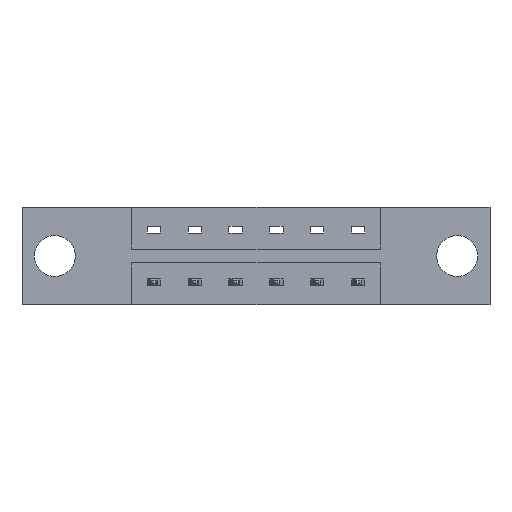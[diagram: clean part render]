
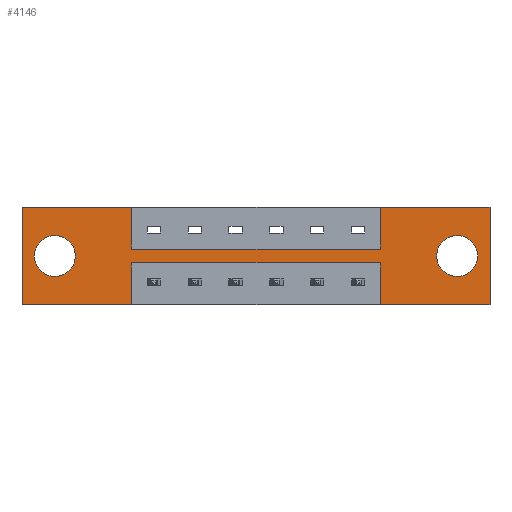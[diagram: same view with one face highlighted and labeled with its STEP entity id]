
A CAD part, front view. The second image highlights one B-rep face of the part: STEP entity #4146.
In plain terms, the highlighted planar face has unit normal (0, -1, 0).
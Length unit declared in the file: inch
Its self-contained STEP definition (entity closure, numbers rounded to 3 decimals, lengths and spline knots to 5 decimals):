
#99 = LINE ( 'NONE', #126, #4949 ) ;
#100 = DIRECTION ( 'NONE',  ( 0., 0., 1. ) ) ;
#126 = CARTESIAN_POINT ( 'NONE',  ( 1.3665, 0., -0.2115 ) ) ;
#155 = DIRECTION ( 'NONE',  ( 0., 0., 1. ) ) ;
#167 = VECTOR ( 'NONE', #100, 39.37008 ) ;
#278 = ORIENTED_EDGE ( 'NONE', *, *, #4959, .T. ) ;
#288 = CARTESIAN_POINT ( 'NONE',  ( 1.3665, 0., 0. ) ) ;
#317 = PLANE ( 'NONE',  #1604 ) ;
#338 = VECTOR ( 'NONE', #7454, 39.37008 ) ;
#372 = EDGE_CURVE ( 'NONE', #6949, #3484, #2396, .T. ) ;
#422 = EDGE_CURVE ( 'NONE', #7205, #1495, #5241, .T. ) ;
#458 = CARTESIAN_POINT ( 'NONE',  ( 0.4175, 0., -0.37 ) ) ;
#490 = EDGE_CURVE ( 'NONE', #2468, #7711, #6305, .T. ) ;
#650 = VERTEX_POINT ( 'NONE', #3517 ) ;
#700 = DIRECTION ( 'NONE',  ( 1., 0., 0. ) ) ;
#738 = EDGE_LOOP ( 'NONE', ( #4732, #3456 ) ) ;
#781 = DIRECTION ( 'NONE',  ( 0., 1., 0. ) ) ;
#785 = LINE ( 'NONE', #6938, #3924 ) ;
#843 = VECTOR ( 'NONE', #6779, 39.37008 ) ;
#920 = VECTOR ( 'NONE', #700, 39.37008 ) ;
#968 = VECTOR ( 'NONE', #1277, 39.37008 ) ;
#1149 = ORIENTED_EDGE ( 'NONE', *, *, #7257, .F. ) ;
#1171 = DIRECTION ( 'NONE',  ( 0., 1., 0. ) ) ;
#1260 = ORIENTED_EDGE ( 'NONE', *, *, #8287, .F. ) ;
#1277 = DIRECTION ( 'NONE',  ( -1., 0., 0. ) ) ;
#1366 = AXIS2_PLACEMENT_3D ( 'NONE', #3649, #3646, #3790 ) ;
#1377 = ORIENTED_EDGE ( 'NONE', *, *, #3852, .F. ) ;
#1420 = EDGE_CURVE ( 'NONE', #1495, #4481, #8238, .T. ) ;
#1432 = DIRECTION ( 'NONE',  ( 1., 0., 0. ) ) ;
#1477 = CARTESIAN_POINT ( 'NONE',  ( 0., 0., -0.37 ) ) ;
#1479 = ORIENTED_EDGE ( 'NONE', *, *, #7361, .F. ) ;
#1495 = VERTEX_POINT ( 'NONE', #5935 ) ;
#1552 = CIRCLE ( 'NONE', #5682, 0.078 ) ;
#1553 = AXIS2_PLACEMENT_3D ( 'NONE', #5091, #1171, #5745 ) ;
#1584 = ORIENTED_EDGE ( 'NONE', *, *, #4797, .F. ) ;
#1604 = AXIS2_PLACEMENT_3D ( 'NONE', #3143, #6990, #3573 ) ;
#1618 = CARTESIAN_POINT ( 'NONE',  ( 0.4175, 0., -0.1585 ) ) ;
#1636 = EDGE_CURVE ( 'NONE', #650, #2468, #7103, .T. ) ;
#1639 = VERTEX_POINT ( 'NONE', #3883 ) ;
#1642 = FACE_BOUND ( 'NONE', #7378, .T. ) ;
#1691 = EDGE_CURVE ( 'NONE', #3484, #6949, #1552, .T. ) ;
#1788 = ORIENTED_EDGE ( 'NONE', *, *, #3382, .F. ) ;
#2017 = CARTESIAN_POINT ( 'NONE',  ( 1.3665, 0., -0.2115 ) ) ;
#2110 = CARTESIAN_POINT ( 'NONE',  ( 0., 0., 0. ) ) ;
#2114 = ORIENTED_EDGE ( 'NONE', *, *, #7131, .F. ) ;
#2246 = AXIS2_PLACEMENT_3D ( 'NONE', #4728, #781, #5379 ) ;
#2396 = CIRCLE ( 'NONE', #1366, 0.078 ) ;
#2468 = VERTEX_POINT ( 'NONE', #288 ) ;
#2552 = VECTOR ( 'NONE', #4674, 39.37008 ) ;
#2641 = VERTEX_POINT ( 'NONE', #2017 ) ;
#2646 = CARTESIAN_POINT ( 'NONE',  ( 0., 0., -0.37 ) ) ;
#2861 = ORIENTED_EDGE ( 'NONE', *, *, #1636, .F. ) ;
#2927 = VERTEX_POINT ( 'NONE', #6254 ) ;
#3143 = CARTESIAN_POINT ( 'NONE',  ( 0., 0., -0.37 ) ) ;
#3242 = VECTOR ( 'NONE', #1432, 39.37008 ) ;
#3321 = CARTESIAN_POINT ( 'NONE',  ( 0., 0., 0. ) ) ;
#3342 = VECTOR ( 'NONE', #3916, 39.37008 ) ;
#3382 = EDGE_CURVE ( 'NONE', #7711, #5149, #7098, .T. ) ;
#3456 = ORIENTED_EDGE ( 'NONE', *, *, #1691, .T. ) ;
#3484 = VERTEX_POINT ( 'NONE', #6794 ) ;
#3517 = CARTESIAN_POINT ( 'NONE',  ( 1.3665, 0., -0.1585 ) ) ;
#3553 = DIRECTION ( 'NONE',  ( 0., 0., -1. ) ) ;
#3573 = DIRECTION ( 'NONE',  ( 0., 0., -1. ) ) ;
#3646 = DIRECTION ( 'NONE',  ( 0., 1., 0. ) ) ;
#3649 = CARTESIAN_POINT ( 'NONE',  ( 1.659, 0., -0.185 ) ) ;
#3655 = ORIENTED_EDGE ( 'NONE', *, *, #422, .F. ) ;
#3754 = ORIENTED_EDGE ( 'NONE', *, *, #490, .F. ) ;
#3790 = DIRECTION ( 'NONE',  ( 0., 0., -1. ) ) ;
#3852 = EDGE_CURVE ( 'NONE', #1639, #6910, #785, .T. ) ;
#3874 = EDGE_LOOP ( 'NONE', ( #1149, #5035, #1788, #3754, #2861, #1260, #1479, #4933, #3655, #2114, #1377, #1584 ) ) ;
#3883 = CARTESIAN_POINT ( 'NONE',  ( 0.4175, 0., -0.2115 ) ) ;
#3916 = DIRECTION ( 'NONE',  ( 0., 0., 1. ) ) ;
#3924 = VECTOR ( 'NONE', #5581, 39.37008 ) ;
#3993 = CARTESIAN_POINT ( 'NONE',  ( 0.4175, 0., -0.1585 ) ) ;
#4102 = LINE ( 'NONE', #6807, #338 ) ;
#4146 = ADVANCED_FACE ( 'NONE', ( #8221, #1642, #5102 ), #317, .T. ) ;
#4168 = CARTESIAN_POINT ( 'NONE',  ( 1.784, 0., 0. ) ) ;
#4269 = LINE ( 'NONE', #7209, #2552 ) ;
#4353 = LINE ( 'NONE', #1618, #843 ) ;
#4481 = VERTEX_POINT ( 'NONE', #8273 ) ;
#4550 = VERTEX_POINT ( 'NONE', #3993 ) ;
#4622 = VECTOR ( 'NONE', #6198, 39.37008 ) ;
#4674 = DIRECTION ( 'NONE',  ( -1., 0., 0. ) ) ;
#4728 = CARTESIAN_POINT ( 'NONE',  ( 0.125, 0., -0.185 ) ) ;
#4732 = ORIENTED_EDGE ( 'NONE', *, *, #372, .T. ) ;
#4797 = EDGE_CURVE ( 'NONE', #2641, #1639, #4102, .T. ) ;
#4933 = ORIENTED_EDGE ( 'NONE', *, *, #1420, .F. ) ;
#4949 = VECTOR ( 'NONE', #155, 39.37008 ) ;
#4959 = EDGE_CURVE ( 'NONE', #2927, #7752, #7568, .T. ) ;
#5035 = ORIENTED_EDGE ( 'NONE', *, *, #5625, .F. ) ;
#5091 = CARTESIAN_POINT ( 'NONE',  ( 0.125, 0., -0.185 ) ) ;
#5102 = FACE_OUTER_BOUND ( 'NONE', #3874, .T. ) ;
#5149 = VERTEX_POINT ( 'NONE', #6553 ) ;
#5241 = LINE ( 'NONE', #8141, #167 ) ;
#5314 = CARTESIAN_POINT ( 'NONE',  ( 0.4175, 0., -0.1585 ) ) ;
#5379 = DIRECTION ( 'NONE',  ( 0., 0., 1. ) ) ;
#5425 = VECTOR ( 'NONE', #3553, 39.37008 ) ;
#5581 = DIRECTION ( 'NONE',  ( 0., 0., -1. ) ) ;
#5625 = EDGE_CURVE ( 'NONE', #5149, #7440, #5976, .T. ) ;
#5682 = AXIS2_PLACEMENT_3D ( 'NONE', #7008, #6991, #6986 ) ;
#5745 = DIRECTION ( 'NONE',  ( 0., 0., 1. ) ) ;
#5850 = CARTESIAN_POINT ( 'NONE',  ( 1.784, 0., 0. ) ) ;
#5935 = CARTESIAN_POINT ( 'NONE',  ( 0., 0., 0. ) ) ;
#5976 = LINE ( 'NONE', #2646, #968 ) ;
#6198 = DIRECTION ( 'NONE',  ( 1., 0., 0. ) ) ;
#6254 = CARTESIAN_POINT ( 'NONE',  ( 0.125, 0., -0.107 ) ) ;
#6305 = LINE ( 'NONE', #3321, #4622 ) ;
#6553 = CARTESIAN_POINT ( 'NONE',  ( 1.784, 0., -0.37 ) ) ;
#6779 = DIRECTION ( 'NONE',  ( 0., 0., -1. ) ) ;
#6794 = CARTESIAN_POINT ( 'NONE',  ( 1.659, 0., -0.263 ) ) ;
#6807 = CARTESIAN_POINT ( 'NONE',  ( 0.4175, 0., -0.2115 ) ) ;
#6910 = VERTEX_POINT ( 'NONE', #458 ) ;
#6938 = CARTESIAN_POINT ( 'NONE',  ( 0.4175, 0., -0.2115 ) ) ;
#6949 = VERTEX_POINT ( 'NONE', #7627 ) ;
#6986 = DIRECTION ( 'NONE',  ( 0., 0., -1. ) ) ;
#6990 = DIRECTION ( 'NONE',  ( 0., -1., 0. ) ) ;
#6991 = DIRECTION ( 'NONE',  ( 0., 1., 0. ) ) ;
#7008 = CARTESIAN_POINT ( 'NONE',  ( 1.659, 0., -0.185 ) ) ;
#7098 = LINE ( 'NONE', #4168, #5425 ) ;
#7103 = LINE ( 'NONE', #7681, #3342 ) ;
#7131 = EDGE_CURVE ( 'NONE', #6910, #7205, #4269, .T. ) ;
#7200 = EDGE_CURVE ( 'NONE', #7752, #2927, #7250, .T. ) ;
#7205 = VERTEX_POINT ( 'NONE', #1477 ) ;
#7209 = CARTESIAN_POINT ( 'NONE',  ( 0., 0., -0.37 ) ) ;
#7223 = ORIENTED_EDGE ( 'NONE', *, *, #7200, .T. ) ;
#7250 = CIRCLE ( 'NONE', #2246, 0.078 ) ;
#7257 = EDGE_CURVE ( 'NONE', #7440, #2641, #99, .T. ) ;
#7361 = EDGE_CURVE ( 'NONE', #4481, #4550, #4353, .T. ) ;
#7378 = EDGE_LOOP ( 'NONE', ( #278, #7223 ) ) ;
#7440 = VERTEX_POINT ( 'NONE', #8046 ) ;
#7454 = DIRECTION ( 'NONE',  ( -1., 0., 0. ) ) ;
#7568 = CIRCLE ( 'NONE', #1553, 0.078 ) ;
#7627 = CARTESIAN_POINT ( 'NONE',  ( 1.659, 0., -0.107 ) ) ;
#7681 = CARTESIAN_POINT ( 'NONE',  ( 1.3665, 0., -0.1585 ) ) ;
#7711 = VERTEX_POINT ( 'NONE', #5850 ) ;
#7752 = VERTEX_POINT ( 'NONE', #8344 ) ;
#7801 = LINE ( 'NONE', #5314, #920 ) ;
#8046 = CARTESIAN_POINT ( 'NONE',  ( 1.3665, 0., -0.37 ) ) ;
#8141 = CARTESIAN_POINT ( 'NONE',  ( 0., 0., 0. ) ) ;
#8221 = FACE_BOUND ( 'NONE', #738, .T. ) ;
#8238 = LINE ( 'NONE', #2110, #3242 ) ;
#8273 = CARTESIAN_POINT ( 'NONE',  ( 0.4175, 0., 0. ) ) ;
#8287 = EDGE_CURVE ( 'NONE', #4550, #650, #7801, .T. ) ;
#8344 = CARTESIAN_POINT ( 'NONE',  ( 0.125, 0., -0.263 ) ) ;
